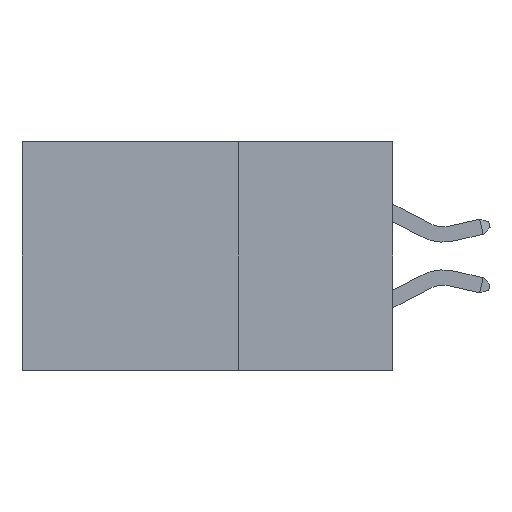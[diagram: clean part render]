
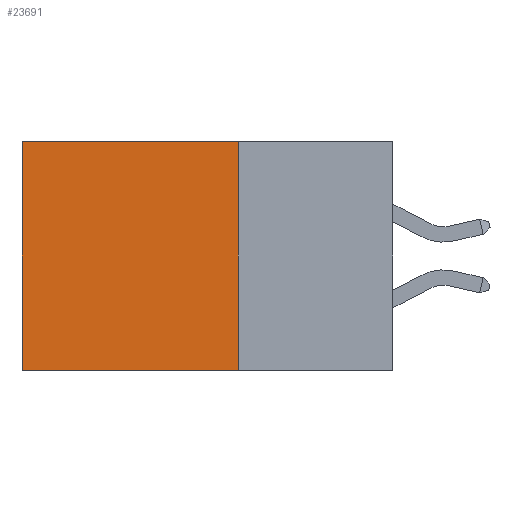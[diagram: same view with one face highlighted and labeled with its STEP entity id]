
A CAD part, left-side view. The second image highlights one B-rep face of the part: STEP entity #23691.
In plain terms, the highlighted planar face has unit normal (-1, 0, 0).
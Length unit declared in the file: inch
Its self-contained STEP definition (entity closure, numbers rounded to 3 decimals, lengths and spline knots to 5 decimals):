
#211 = VERTEX_POINT ( 'NONE', #5482 ) ;
#994 = FACE_OUTER_BOUND ( 'NONE', #20655, .T. ) ;
#3669 = CARTESIAN_POINT ( 'NONE',  ( 0.2875, 0.6, 0. ) ) ;
#4154 = VECTOR ( 'NONE', #13737, 39.37008 ) ;
#4182 = CARTESIAN_POINT ( 'NONE',  ( 0.2875, 0.6, -0.37 ) ) ;
#4233 = VECTOR ( 'NONE', #14699, 39.37008 ) ;
#4582 = VERTEX_POINT ( 'NONE', #21872 ) ;
#4751 = LINE ( 'NONE', #18891, #4154 ) ;
#4914 = VERTEX_POINT ( 'NONE', #4182 ) ;
#5482 = CARTESIAN_POINT ( 'NONE',  ( 0.2875, 0.25, -0.37 ) ) ;
#5524 = VECTOR ( 'NONE', #18888, 39.37008 ) ;
#5654 = PLANE ( 'NONE',  #13941 ) ;
#5743 = ORIENTED_EDGE ( 'NONE', *, *, #21111, .F. ) ;
#6982 = LINE ( 'NONE', #3669, #5524 ) ;
#7290 = LINE ( 'NONE', #8856, #18941 ) ;
#7531 = EDGE_CURVE ( 'NONE', #4582, #4914, #6982, .T. ) ;
#8856 = CARTESIAN_POINT ( 'NONE',  ( 0.2875, 0.25, 0. ) ) ;
#10645 = ORIENTED_EDGE ( 'NONE', *, *, #16186, .F. ) ;
#11387 = DIRECTION ( 'NONE',  ( 0., 0., -1. ) ) ;
#11852 = LINE ( 'NONE', #20149, #4233 ) ;
#12699 = DIRECTION ( 'NONE',  ( 0., 1., 0. ) ) ;
#13737 = DIRECTION ( 'NONE',  ( 0., 1., 0. ) ) ;
#13941 = AXIS2_PLACEMENT_3D ( 'NONE', #20567, #15034, #11387 ) ;
#14699 = DIRECTION ( 'NONE',  ( 0., 0., -1. ) ) ;
#15034 = DIRECTION ( 'NONE',  ( 1., 0., 0. ) ) ;
#15723 = CARTESIAN_POINT ( 'NONE',  ( 0.2875, 0.25, 0. ) ) ;
#16186 = EDGE_CURVE ( 'NONE', #211, #4914, #4751, .T. ) ;
#16348 = ORIENTED_EDGE ( 'NONE', *, *, #17668, .T. ) ;
#17668 = EDGE_CURVE ( 'NONE', #18672, #4582, #7290, .T. ) ;
#18672 = VERTEX_POINT ( 'NONE', #15723 ) ;
#18888 = DIRECTION ( 'NONE',  ( 0., 0., -1. ) ) ;
#18891 = CARTESIAN_POINT ( 'NONE',  ( 0.2875, 0.25, -0.37 ) ) ;
#18941 = VECTOR ( 'NONE', #12699, 39.37008 ) ;
#19701 = ORIENTED_EDGE ( 'NONE', *, *, #7531, .T. ) ;
#20149 = CARTESIAN_POINT ( 'NONE',  ( 0.2875, 0.25, 0. ) ) ;
#20567 = CARTESIAN_POINT ( 'NONE',  ( 0.2875, 0.25, 0. ) ) ;
#20655 = EDGE_LOOP ( 'NONE', ( #19701, #10645, #5743, #16348 ) ) ;
#21111 = EDGE_CURVE ( 'NONE', #18672, #211, #11852, .T. ) ;
#21872 = CARTESIAN_POINT ( 'NONE',  ( 0.2875, 0.6, 0. ) ) ;
#23691 = ADVANCED_FACE ( 'NONE', ( #994 ), #5654, .F. ) ;
